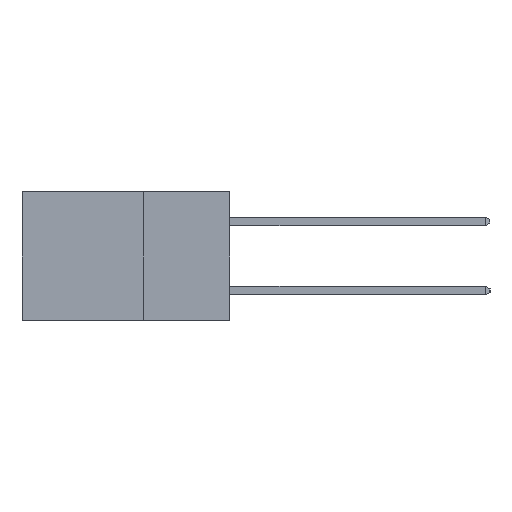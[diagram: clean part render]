
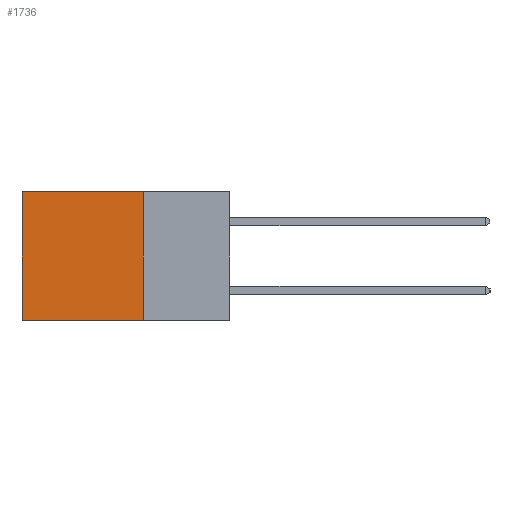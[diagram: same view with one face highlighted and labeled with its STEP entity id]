
A CAD part, left-side view. The second image highlights one B-rep face of the part: STEP entity #1736.
In plain terms, the highlighted planar face has unit normal (-1, 0, 0).
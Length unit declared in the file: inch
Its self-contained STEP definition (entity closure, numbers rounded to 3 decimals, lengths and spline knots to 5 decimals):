
#224 = CARTESIAN_POINT ( 'NONE',  ( 0.2615, 0.25, 0. ) ) ;
#698 = LINE ( 'NONE', #7577, #11245 ) ;
#943 = VECTOR ( 'NONE', #2261, 39.37008 ) ;
#1070 = CARTESIAN_POINT ( 'NONE',  ( 0.2615, 0.25, -0.37 ) ) ;
#1736 = ADVANCED_FACE ( 'NONE', ( #1998 ), #9042, .F. ) ;
#1998 = FACE_OUTER_BOUND ( 'NONE', #6608, .T. ) ;
#2261 = DIRECTION ( 'NONE',  ( 0., 1., 0. ) ) ;
#2325 = CARTESIAN_POINT ( 'NONE',  ( 0.2615, 0.25, -0.37 ) ) ;
#2573 = EDGE_CURVE ( 'NONE', #8639, #6694, #10609, .T. ) ;
#3542 = CARTESIAN_POINT ( 'NONE',  ( 0.2615, 0.6, 0. ) ) ;
#3882 = ORIENTED_EDGE ( 'NONE', *, *, #11072, .F. ) ;
#4215 = DIRECTION ( 'NONE',  ( 0., 0., -1. ) ) ;
#4231 = CARTESIAN_POINT ( 'NONE',  ( 0.2615, 0.25, -0.37 ) ) ;
#5689 = CARTESIAN_POINT ( 'NONE',  ( 0.2615, 0.25, -0.37 ) ) ;
#6153 = VERTEX_POINT ( 'NONE', #1070 ) ;
#6248 = CARTESIAN_POINT ( 'NONE',  ( 0.2615, 0.6, -0.37 ) ) ;
#6345 = LINE ( 'NONE', #2325, #943 ) ;
#6608 = EDGE_LOOP ( 'NONE', ( #7782, #3882, #10316, #9388 ) ) ;
#6694 = VERTEX_POINT ( 'NONE', #6248 ) ;
#7303 = VECTOR ( 'NONE', #4215, 39.37008 ) ;
#7386 = DIRECTION ( 'NONE',  ( 0., 1., 0. ) ) ;
#7577 = CARTESIAN_POINT ( 'NONE',  ( 0.2615, 0.25, 0. ) ) ;
#7782 = ORIENTED_EDGE ( 'NONE', *, *, #2573, .T. ) ;
#7816 = VECTOR ( 'NONE', #11526, 39.37008 ) ;
#8312 = EDGE_CURVE ( 'NONE', #11542, #8639, #698, .T. ) ;
#8639 = VERTEX_POINT ( 'NONE', #3542 ) ;
#9042 = PLANE ( 'NONE',  #11863 ) ;
#9388 = ORIENTED_EDGE ( 'NONE', *, *, #8312, .T. ) ;
#9618 = EDGE_CURVE ( 'NONE', #11542, #6153, #9781, .T. ) ;
#9781 = LINE ( 'NONE', #4231, #7303 ) ;
#10316 = ORIENTED_EDGE ( 'NONE', *, *, #9618, .F. ) ;
#10609 = LINE ( 'NONE', #11632, #7816 ) ;
#11072 = EDGE_CURVE ( 'NONE', #6153, #6694, #6345, .T. ) ;
#11245 = VECTOR ( 'NONE', #7386, 39.37008 ) ;
#11526 = DIRECTION ( 'NONE',  ( 0., 0., -1. ) ) ;
#11542 = VERTEX_POINT ( 'NONE', #224 ) ;
#11632 = CARTESIAN_POINT ( 'NONE',  ( 0.2615, 0.6, -0.37 ) ) ;
#11863 = AXIS2_PLACEMENT_3D ( 'NONE', #5689, #12673, #12535 ) ;
#12535 = DIRECTION ( 'NONE',  ( 0., 0., -1. ) ) ;
#12673 = DIRECTION ( 'NONE',  ( 1., 0., 0. ) ) ;
